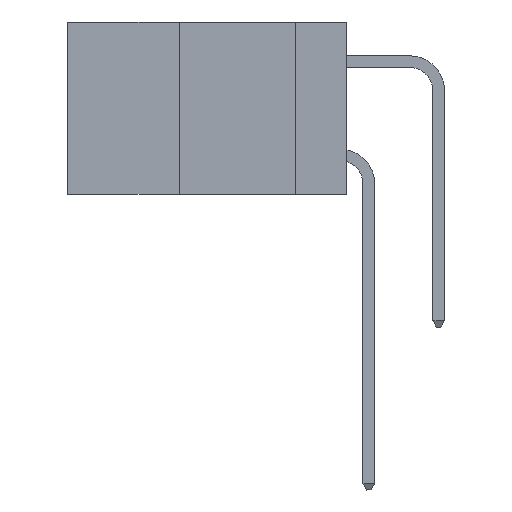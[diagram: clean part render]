
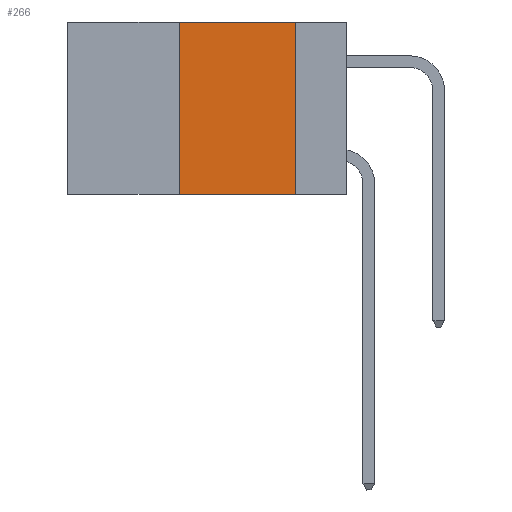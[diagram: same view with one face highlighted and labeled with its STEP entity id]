
A CAD part, left-side view. The second image highlights one B-rep face of the part: STEP entity #266.
In plain terms, the highlighted planar face has unit normal (-1, 0, 0).
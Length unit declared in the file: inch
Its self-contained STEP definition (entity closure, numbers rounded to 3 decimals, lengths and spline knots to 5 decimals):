
#266 = ADVANCED_FACE ( 'NONE', ( #765 ), #26119, .F. ) ;
#376 = VECTOR ( 'NONE', #8142, 39.37008 ) ;
#569 = VECTOR ( 'NONE', #35161, 39.37008 ) ;
#765 = FACE_OUTER_BOUND ( 'NONE', #28073, .T. ) ;
#3312 = VERTEX_POINT ( 'NONE', #18952 ) ;
#4076 = CARTESIAN_POINT ( 'NONE',  ( 0., 0.11, -0.37 ) ) ;
#5342 = CARTESIAN_POINT ( 'NONE',  ( 0., 0.6, 0. ) ) ;
#5738 = DIRECTION ( 'NONE',  ( 0., 0., 1. ) ) ;
#7191 = DIRECTION ( 'NONE',  ( 1., 0., 0. ) ) ;
#8142 = DIRECTION ( 'NONE',  ( 0., -1., 0. ) ) ;
#8656 = LINE ( 'NONE', #22113, #23139 ) ;
#9556 = CARTESIAN_POINT ( 'NONE',  ( 0., 0.6, -0.37 ) ) ;
#9563 = EDGE_CURVE ( 'NONE', #3312, #23567, #8656, .T. ) ;
#10343 = CARTESIAN_POINT ( 'NONE',  ( 0., 0.11, 0. ) ) ;
#13293 = VECTOR ( 'NONE', #25825, 39.37008 ) ;
#14531 = EDGE_CURVE ( 'NONE', #23567, #24041, #22294, .T. ) ;
#16118 = LINE ( 'NONE', #21640, #569 ) ;
#16883 = ORIENTED_EDGE ( 'NONE', *, *, #24158, .F. ) ;
#18952 = CARTESIAN_POINT ( 'NONE',  ( 0., 0.36, -0.37 ) ) ;
#21640 = CARTESIAN_POINT ( 'NONE',  ( 0., 0.11, 0. ) ) ;
#22113 = CARTESIAN_POINT ( 'NONE',  ( 0., 0.36, 0. ) ) ;
#22294 = LINE ( 'NONE', #5342, #376 ) ;
#23139 = VECTOR ( 'NONE', #5738, 39.37008 ) ;
#23530 = CARTESIAN_POINT ( 'NONE',  ( 0., 0.6, 0. ) ) ;
#23567 = VERTEX_POINT ( 'NONE', #29699 ) ;
#24041 = VERTEX_POINT ( 'NONE', #10343 ) ;
#24093 = ORIENTED_EDGE ( 'NONE', *, *, #14531, .F. ) ;
#24158 = EDGE_CURVE ( 'NONE', #24041, #26570, #16118, .T. ) ;
#25825 = DIRECTION ( 'NONE',  ( 0., -1., 0. ) ) ;
#26119 = PLANE ( 'NONE',  #31757 ) ;
#26236 = DIRECTION ( 'NONE',  ( 0., 0., -1. ) ) ;
#26570 = VERTEX_POINT ( 'NONE', #4076 ) ;
#28073 = EDGE_LOOP ( 'NONE', ( #16883, #24093, #31271, #32946 ) ) ;
#28439 = EDGE_CURVE ( 'NONE', #3312, #26570, #29414, .T. ) ;
#29414 = LINE ( 'NONE', #9556, #13293 ) ;
#29699 = CARTESIAN_POINT ( 'NONE',  ( 0., 0.36, 0. ) ) ;
#31271 = ORIENTED_EDGE ( 'NONE', *, *, #9563, .F. ) ;
#31757 = AXIS2_PLACEMENT_3D ( 'NONE', #23530, #7191, #26236 ) ;
#32946 = ORIENTED_EDGE ( 'NONE', *, *, #28439, .T. ) ;
#35161 = DIRECTION ( 'NONE',  ( 0., 0., -1. ) ) ;
